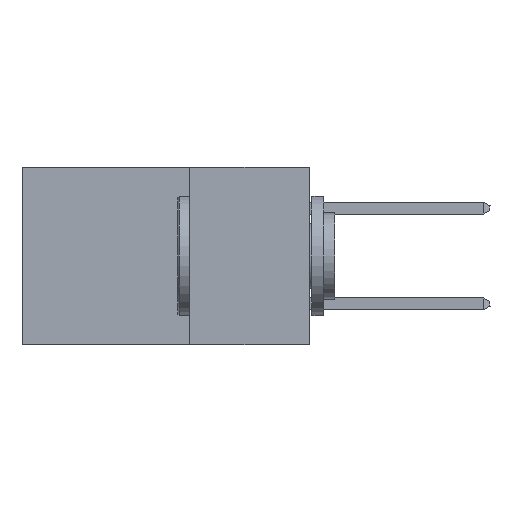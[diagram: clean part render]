
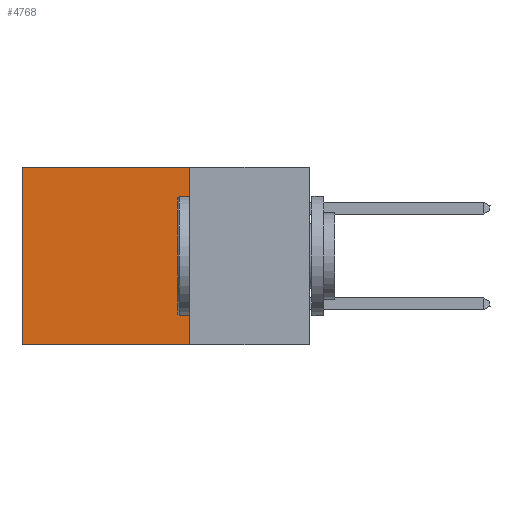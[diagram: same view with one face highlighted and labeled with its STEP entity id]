
A CAD part, left-side view. The second image highlights one B-rep face of the part: STEP entity #4768.
In plain terms, the highlighted planar face has unit normal (-1, 0, 0).
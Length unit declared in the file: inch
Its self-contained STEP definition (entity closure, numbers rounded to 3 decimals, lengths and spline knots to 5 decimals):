
#148 = DIRECTION ( 'NONE',  ( 0., 0., -1. ) ) ;
#161 = ORIENTED_EDGE ( 'NONE', *, *, #16528, .F. ) ;
#596 = DIRECTION ( 'NONE',  ( 0., 1., 0. ) ) ;
#4748 = DIRECTION ( 'NONE',  ( 1., 0., 0. ) ) ;
#4768 = ADVANCED_FACE ( 'NONE', ( #15939 ), #11785, .F. ) ;
#5416 = EDGE_CURVE ( 'NONE', #20979, #10789, #16996, .T. ) ;
#5418 = DIRECTION ( 'NONE',  ( 0., 1., 0. ) ) ;
#8911 = DIRECTION ( 'NONE',  ( 0., 0., -1. ) ) ;
#10789 = VERTEX_POINT ( 'NONE', #21180 ) ;
#11124 = CARTESIAN_POINT ( 'NONE',  ( 0.2875, 0.6, 0. ) ) ;
#11785 = PLANE ( 'NONE',  #21998 ) ;
#11960 = CARTESIAN_POINT ( 'NONE',  ( 0.2875, 0.25, 0. ) ) ;
#12965 = VECTOR ( 'NONE', #8911, 39.37008 ) ;
#13436 = EDGE_LOOP ( 'NONE', ( #20143, #161, #29533, #15154 ) ) ;
#15154 = ORIENTED_EDGE ( 'NONE', *, *, #21341, .T. ) ;
#15939 = FACE_OUTER_BOUND ( 'NONE', #13436, .T. ) ;
#16528 = EDGE_CURVE ( 'NONE', #10789, #29284, #28925, .T. ) ;
#16996 = LINE ( 'NONE', #11960, #22559 ) ;
#18337 = CARTESIAN_POINT ( 'NONE',  ( 0.2875, 0.6, 0. ) ) ;
#18452 = VERTEX_POINT ( 'NONE', #11124 ) ;
#18909 = CARTESIAN_POINT ( 'NONE',  ( 0.2875, 0.25, 0. ) ) ;
#19604 = CARTESIAN_POINT ( 'NONE',  ( 0.2875, 0.25, 0. ) ) ;
#20026 = LINE ( 'NONE', #18337, #12965 ) ;
#20143 = ORIENTED_EDGE ( 'NONE', *, *, #27173, .T. ) ;
#20775 = CARTESIAN_POINT ( 'NONE',  ( 0.2875, 0.25, 0. ) ) ;
#20979 = VERTEX_POINT ( 'NONE', #20775 ) ;
#21180 = CARTESIAN_POINT ( 'NONE',  ( 0.2875, 0.25, -0.37 ) ) ;
#21304 = DIRECTION ( 'NONE',  ( 0., 0., -1. ) ) ;
#21341 = EDGE_CURVE ( 'NONE', #20979, #18452, #21462, .T. ) ;
#21462 = LINE ( 'NONE', #19604, #26881 ) ;
#21998 = AXIS2_PLACEMENT_3D ( 'NONE', #18909, #4748, #21304 ) ;
#22096 = VECTOR ( 'NONE', #596, 39.37008 ) ;
#22559 = VECTOR ( 'NONE', #148, 39.37008 ) ;
#26881 = VECTOR ( 'NONE', #5418, 39.37008 ) ;
#27173 = EDGE_CURVE ( 'NONE', #18452, #29284, #20026, .T. ) ;
#28723 = CARTESIAN_POINT ( 'NONE',  ( 0.2875, 0.25, -0.37 ) ) ;
#28925 = LINE ( 'NONE', #28723, #22096 ) ;
#29072 = CARTESIAN_POINT ( 'NONE',  ( 0.2875, 0.6, -0.37 ) ) ;
#29284 = VERTEX_POINT ( 'NONE', #29072 ) ;
#29533 = ORIENTED_EDGE ( 'NONE', *, *, #5416, .F. ) ;
